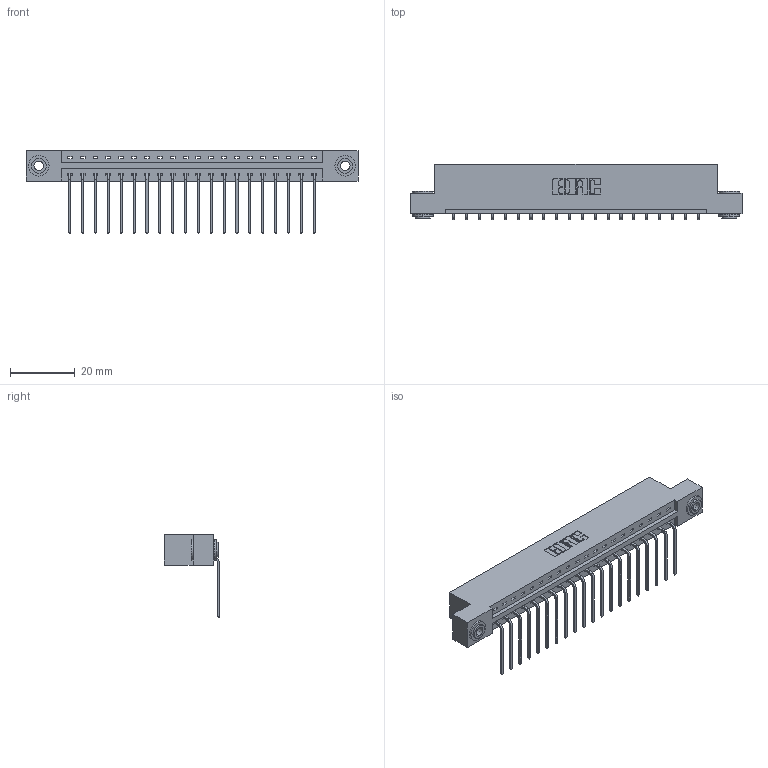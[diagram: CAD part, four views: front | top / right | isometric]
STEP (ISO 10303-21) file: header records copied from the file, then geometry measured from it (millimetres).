
FILE_DESCRIPTION (( 'STEP AP203' ), '1' );
FILE_NAME ('337-020-559-103.STEP', '2018-08-05T10:31:45', ( '' ), ( '' ), 'SwSTEP 2.0', 'SolidWorks 2016', '' );
FILE_SCHEMA (( 'CONFIG_CONTROL_DESIGN' ));
Length unit declared in the file: inch
Products named in the file (4): 345-250-002_345-250-002-102; 337-020-559-103; 337 Part_Flush Mounting Lugs - 0.156 Dia-TH; 345-292-001_558 559 Tail - 1
Assembly tree (23 placements, depth 2):
  337-020-559-103
    337 Part_Flush Mounting Lugs - 0.156 Dia-TH
    345-292-001_558 559 Tail - 1  x20
    345-250-002_345-250-002-102  x2
Bounding box: 102.26 x 17.09 x 25.53 mm (x, y, z)
Volume: 10439 mm3; surface area: 11307.1 mm2
Topology: 23 solids, 23 shells, 1432 faces, 4267 edges, 2814 vertices
Faces by surface type: plane 1040, cylinder 384, cone 8
Entity records: 18446 total; most frequent: CARTESIAN_POINT 3189, ORIENTED_EDGE 3138, DIRECTION 2763, EDGE_CURVE 1569, LINE 1417, VECTOR 1417, VERTEX_POINT 1042, AXIS2_PLACEMENT_3D 673
